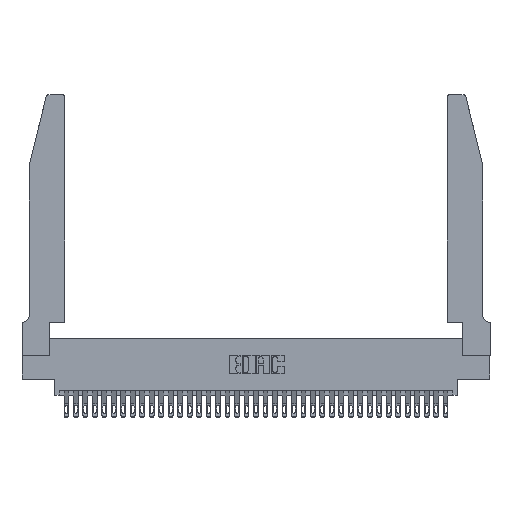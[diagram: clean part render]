
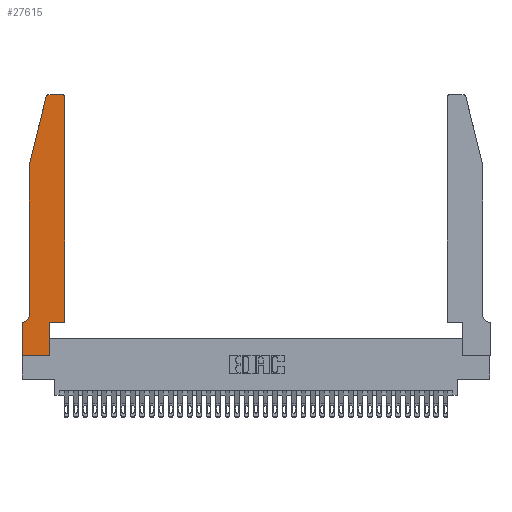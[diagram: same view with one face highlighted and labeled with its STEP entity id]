
A CAD part, top view. The second image highlights one B-rep face of the part: STEP entity #27615.
In plain terms, the highlighted planar face has unit normal (0, 0, 1).
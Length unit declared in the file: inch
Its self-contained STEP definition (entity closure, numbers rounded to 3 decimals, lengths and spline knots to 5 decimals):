
#539 = VERTEX_POINT ( 'NONE', #25779 ) ;
#569 = DIRECTION ( 'NONE',  ( 1., 0., 0. ) ) ;
#1802 = CARTESIAN_POINT ( 'NONE',  ( 0.2865, 0.35, 0.37 ) ) ;
#2688 = LINE ( 'NONE', #5109, #35754 ) ;
#2816 = CARTESIAN_POINT ( 'NONE',  ( 0.0755, 0.42, 0.37 ) ) ;
#3358 = CARTESIAN_POINT ( 'NONE',  ( 0.0055, 0.35, 0.37 ) ) ;
#3401 = EDGE_CURVE ( 'NONE', #27522, #19616, #34444, .T. ) ;
#3596 = DIRECTION ( 'NONE',  ( 1., 0., 0. ) ) ;
#3833 = ORIENTED_EDGE ( 'NONE', *, *, #3401, .T. ) ;
#4087 = AXIS2_PLACEMENT_3D ( 'NONE', #29067, #26707, #3596 ) ;
#4812 = EDGE_CURVE ( 'NONE', #35057, #5215, #34341, .T. ) ;
#5036 = EDGE_CURVE ( 'NONE', #9112, #9668, #8923, .T. ) ;
#5109 = CARTESIAN_POINT ( 'NONE',  ( 0.2605, 2.75, 0.37 ) ) ;
#5215 = VERTEX_POINT ( 'NONE', #33788 ) ;
#5528 = CARTESIAN_POINT ( 'NONE',  ( 0.0755, 2., 0.37 ) ) ;
#5679 = EDGE_CURVE ( 'NONE', #9668, #27522, #26646, .T. ) ;
#6165 = ORIENTED_EDGE ( 'NONE', *, *, #12451, .T. ) ;
#7335 = CARTESIAN_POINT ( 'NONE',  ( 0.284, 2.75, 0.37 ) ) ;
#7738 = PLANE ( 'NONE',  #23370 ) ;
#8718 = ORIENTED_EDGE ( 'NONE', *, *, #14223, .T. ) ;
#8923 = CIRCLE ( 'NONE', #4087, 0.03 ) ;
#9112 = VERTEX_POINT ( 'NONE', #7335 ) ;
#9668 = VERTEX_POINT ( 'NONE', #22033 ) ;
#10435 = EDGE_CURVE ( 'NONE', #539, #35057, #30526, .T. ) ;
#11641 = VERTEX_POINT ( 'NONE', #29027 ) ;
#11768 = EDGE_CURVE ( 'NONE', #12409, #539, #13186, .T. ) ;
#12238 = VERTEX_POINT ( 'NONE', #3358 ) ;
#12409 = VERTEX_POINT ( 'NONE', #13002 ) ;
#12451 = EDGE_CURVE ( 'NONE', #22068, #9112, #2688, .T. ) ;
#13002 = CARTESIAN_POINT ( 'NONE',  ( 0., 0., 0.37 ) ) ;
#13186 = LINE ( 'NONE', #26731, #27726 ) ;
#13324 = DIRECTION ( 'NONE',  ( 0., 0., 1. ) ) ;
#13481 = CARTESIAN_POINT ( 'NONE',  ( 0.2865, 0.35, 0.37 ) ) ;
#14223 = EDGE_CURVE ( 'NONE', #5215, #11641, #33454, .T. ) ;
#14471 = EDGE_CURVE ( 'NONE', #12238, #27463, #22117, .T. ) ;
#14791 = DIRECTION ( 'NONE',  ( 0., -1., 0. ) ) ;
#15191 = CARTESIAN_POINT ( 'NONE',  ( 0., 0., 0.37 ) ) ;
#15263 = CARTESIAN_POINT ( 'NONE',  ( 0.4205, 2.75, 0.37 ) ) ;
#15514 = DIRECTION ( 'NONE',  ( 1., 0., 0. ) ) ;
#16235 = DIRECTION ( 'NONE',  ( 1., 0., 0. ) ) ;
#16579 = ORIENTED_EDGE ( 'NONE', *, *, #5036, .T. ) ;
#16611 = ORIENTED_EDGE ( 'NONE', *, *, #21216, .T. ) ;
#16728 = ORIENTED_EDGE ( 'NONE', *, *, #11768, .T. ) ;
#18039 = VECTOR ( 'NONE', #19552, 39.37008 ) ;
#18294 = ORIENTED_EDGE ( 'NONE', *, *, #4812, .T. ) ;
#18851 = DIRECTION ( 'NONE',  ( 0., 0., -1. ) ) ;
#19075 = DIRECTION ( 'NONE',  ( 0., 1., 0. ) ) ;
#19298 = VECTOR ( 'NONE', #14791, 39.37008 ) ;
#19552 = DIRECTION ( 'NONE',  ( -1., 0., 0. ) ) ;
#19616 = VERTEX_POINT ( 'NONE', #2816 ) ;
#20922 = EDGE_LOOP ( 'NONE', ( #6165, #16579, #25110, #3833, #16611, #31466, #36671, #16728, #34354, #18294, #8718, #32084 ) ) ;
#21080 = CARTESIAN_POINT ( 'NONE',  ( 0.4505, 0.35, 0.37 ) ) ;
#21216 = EDGE_CURVE ( 'NONE', #19616, #12238, #35573, .T. ) ;
#21704 = DIRECTION ( 'NONE',  ( 0., 1., 0. ) ) ;
#21917 = VECTOR ( 'NONE', #19075, 39.37008 ) ;
#22033 = CARTESIAN_POINT ( 'NONE',  ( 0.25487, 2.72718, 0.37 ) ) ;
#22068 = VERTEX_POINT ( 'NONE', #15263 ) ;
#22117 = LINE ( 'NONE', #25237, #18039 ) ;
#22146 = DIRECTION ( 'NONE',  ( -1., 0., 0. ) ) ;
#22778 = EDGE_CURVE ( 'NONE', #11641, #22068, #35489, .T. ) ;
#23053 = AXIS2_PLACEMENT_3D ( 'NONE', #24579, #13324, #16235 ) ;
#23370 = AXIS2_PLACEMENT_3D ( 'NONE', #31333, #36729, #31089 ) ;
#23982 = DIRECTION ( 'NONE',  ( 0., -1., 0. ) ) ;
#24579 = CARTESIAN_POINT ( 'NONE',  ( 0.4205, 2.72, 0.37 ) ) ;
#24864 = VECTOR ( 'NONE', #21704, 39.37008 ) ;
#25110 = ORIENTED_EDGE ( 'NONE', *, *, #5679, .T. ) ;
#25132 = DIRECTION ( 'NONE',  ( -0.239, -0.971, 0. ) ) ;
#25237 = CARTESIAN_POINT ( 'NONE',  ( 0.0755, 0.35, 0.37 ) ) ;
#25779 = CARTESIAN_POINT ( 'NONE',  ( 0.2865, 0., 0.37 ) ) ;
#26592 = FACE_OUTER_BOUND ( 'NONE', #20922, .T. ) ;
#26646 = LINE ( 'NONE', #33589, #30281 ) ;
#26707 = DIRECTION ( 'NONE',  ( 0., 0., 1. ) ) ;
#26731 = CARTESIAN_POINT ( 'NONE',  ( 0., 0., 0.37 ) ) ;
#26790 = CARTESIAN_POINT ( 'NONE',  ( 0., 0.35, 0.37 ) ) ;
#27008 = LINE ( 'NONE', #15191, #19298 ) ;
#27234 = VECTOR ( 'NONE', #23982, 39.37008 ) ;
#27436 = CARTESIAN_POINT ( 'NONE',  ( 0.0755, 2., 0.37 ) ) ;
#27463 = VERTEX_POINT ( 'NONE', #26790 ) ;
#27522 = VERTEX_POINT ( 'NONE', #27436 ) ;
#27615 = ADVANCED_FACE ( 'NONE', ( #26592 ), #7738, .T. ) ;
#27726 = VECTOR ( 'NONE', #569, 39.37008 ) ;
#28480 = EDGE_CURVE ( 'NONE', #27463, #12409, #27008, .T. ) ;
#29027 = CARTESIAN_POINT ( 'NONE',  ( 0.4505, 2.72, 0.37 ) ) ;
#29067 = CARTESIAN_POINT ( 'NONE',  ( 0.284, 2.72, 0.37 ) ) ;
#30281 = VECTOR ( 'NONE', #25132, 39.37008 ) ;
#30526 = LINE ( 'NONE', #1802, #21917 ) ;
#30887 = CARTESIAN_POINT ( 'NONE',  ( 0.0055, 0.42, 0.37 ) ) ;
#31089 = DIRECTION ( 'NONE',  ( 1., 0., 0. ) ) ;
#31242 = DIRECTION ( 'NONE',  ( -1., 0., 0. ) ) ;
#31272 = AXIS2_PLACEMENT_3D ( 'NONE', #30887, #18851, #22146 ) ;
#31333 = CARTESIAN_POINT ( 'NONE',  ( 0., 0.35, 0.37 ) ) ;
#31466 = ORIENTED_EDGE ( 'NONE', *, *, #14471, .T. ) ;
#32084 = ORIENTED_EDGE ( 'NONE', *, *, #22778, .T. ) ;
#33190 = CARTESIAN_POINT ( 'NONE',  ( 0.4505, 0.35, 0.37 ) ) ;
#33454 = LINE ( 'NONE', #33190, #24864 ) ;
#33589 = CARTESIAN_POINT ( 'NONE',  ( 0.0755, 2., 0.37 ) ) ;
#33788 = CARTESIAN_POINT ( 'NONE',  ( 0.4505, 0.35, 0.37 ) ) ;
#34341 = LINE ( 'NONE', #21080, #36588 ) ;
#34354 = ORIENTED_EDGE ( 'NONE', *, *, #10435, .T. ) ;
#34444 = LINE ( 'NONE', #5528, #27234 ) ;
#35057 = VERTEX_POINT ( 'NONE', #13481 ) ;
#35489 = CIRCLE ( 'NONE', #23053, 0.03 ) ;
#35573 = CIRCLE ( 'NONE', #31272, 0.07 ) ;
#35754 = VECTOR ( 'NONE', #31242, 39.37008 ) ;
#36588 = VECTOR ( 'NONE', #15514, 39.37008 ) ;
#36671 = ORIENTED_EDGE ( 'NONE', *, *, #28480, .T. ) ;
#36729 = DIRECTION ( 'NONE',  ( 0., 0., 1. ) ) ;
